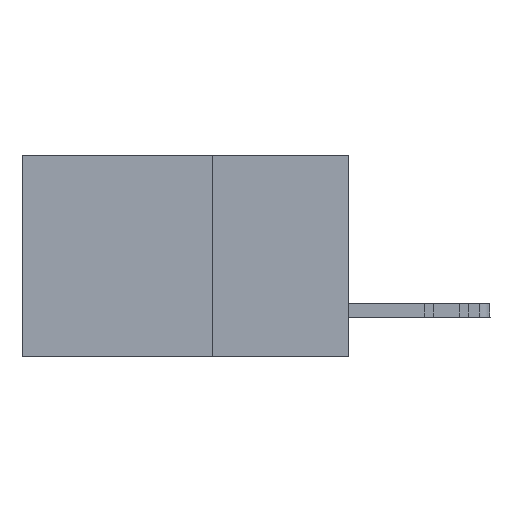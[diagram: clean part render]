
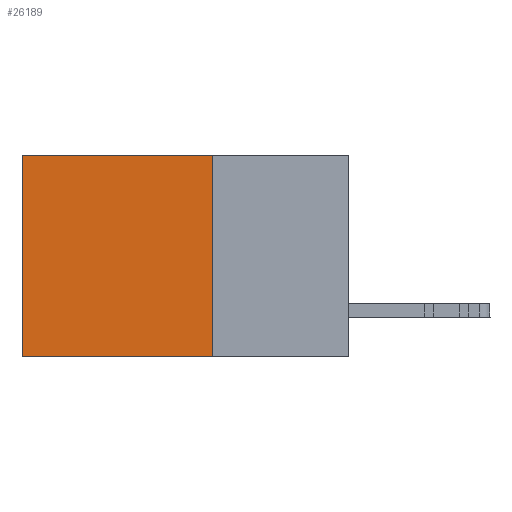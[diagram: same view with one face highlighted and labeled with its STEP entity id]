
A CAD part, left-side view. The second image highlights one B-rep face of the part: STEP entity #26189.
In plain terms, the highlighted planar face has unit normal (-1, 0, 0).
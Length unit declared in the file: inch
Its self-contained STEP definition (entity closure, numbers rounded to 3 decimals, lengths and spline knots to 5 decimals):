
#1349 = CARTESIAN_POINT ( 'NONE',  ( 0.298, 0.25, 0. ) ) ;
#1889 = EDGE_LOOP ( 'NONE', ( #20423, #2235, #6532, #2940 ) ) ;
#2235 = ORIENTED_EDGE ( 'NONE', *, *, #8712, .F. ) ;
#2940 = ORIENTED_EDGE ( 'NONE', *, *, #25579, .T. ) ;
#3675 = CARTESIAN_POINT ( 'NONE',  ( 0.298, 0.25, -0.37 ) ) ;
#4460 = CARTESIAN_POINT ( 'NONE',  ( 0.298, 0.6, -0.37 ) ) ;
#6532 = ORIENTED_EDGE ( 'NONE', *, *, #32531, .F. ) ;
#7190 = VERTEX_POINT ( 'NONE', #3675 ) ;
#8154 = DIRECTION ( 'NONE',  ( 1., 0., 0. ) ) ;
#8712 = EDGE_CURVE ( 'NONE', #7190, #27572, #20520, .T. ) ;
#9726 = LINE ( 'NONE', #11875, #25580 ) ;
#11482 = DIRECTION ( 'NONE',  ( 0., 1., 0. ) ) ;
#11875 = CARTESIAN_POINT ( 'NONE',  ( 0.298, 0.25, 0. ) ) ;
#11962 = LINE ( 'NONE', #22160, #31171 ) ;
#13030 = VECTOR ( 'NONE', #22330, 39.37008 ) ;
#13835 = DIRECTION ( 'NONE',  ( 0., 0., -1. ) ) ;
#18341 = DIRECTION ( 'NONE',  ( 0., 0., -1. ) ) ;
#20423 = ORIENTED_EDGE ( 'NONE', *, *, #31381, .T. ) ;
#20520 = LINE ( 'NONE', #30653, #24251 ) ;
#20851 = CARTESIAN_POINT ( 'NONE',  ( 0.298, 0.25, 0. ) ) ;
#22160 = CARTESIAN_POINT ( 'NONE',  ( 0.298, 0.25, 0. ) ) ;
#22330 = DIRECTION ( 'NONE',  ( 0., 0., -1. ) ) ;
#24136 = VERTEX_POINT ( 'NONE', #1349 ) ;
#24251 = VECTOR ( 'NONE', #11482, 39.37008 ) ;
#25579 = EDGE_CURVE ( 'NONE', #24136, #32953, #9726, .T. ) ;
#25580 = VECTOR ( 'NONE', #32199, 39.37008 ) ;
#25834 = PLANE ( 'NONE',  #27120 ) ;
#26189 = ADVANCED_FACE ( 'NONE', ( #27832 ), #25834, .F. ) ;
#27120 = AXIS2_PLACEMENT_3D ( 'NONE', #20851, #8154, #18341 ) ;
#27572 = VERTEX_POINT ( 'NONE', #4460 ) ;
#27832 = FACE_OUTER_BOUND ( 'NONE', #1889, .T. ) ;
#30653 = CARTESIAN_POINT ( 'NONE',  ( 0.298, 0.25, -0.37 ) ) ;
#30913 = CARTESIAN_POINT ( 'NONE',  ( 0.298, 0.6, 0. ) ) ;
#31171 = VECTOR ( 'NONE', #13835, 39.37008 ) ;
#31381 = EDGE_CURVE ( 'NONE', #32953, #27572, #32970, .T. ) ;
#31945 = CARTESIAN_POINT ( 'NONE',  ( 0.298, 0.6, 0. ) ) ;
#32199 = DIRECTION ( 'NONE',  ( 0., 1., 0. ) ) ;
#32531 = EDGE_CURVE ( 'NONE', #24136, #7190, #11962, .T. ) ;
#32953 = VERTEX_POINT ( 'NONE', #31945 ) ;
#32970 = LINE ( 'NONE', #30913, #13030 ) ;
